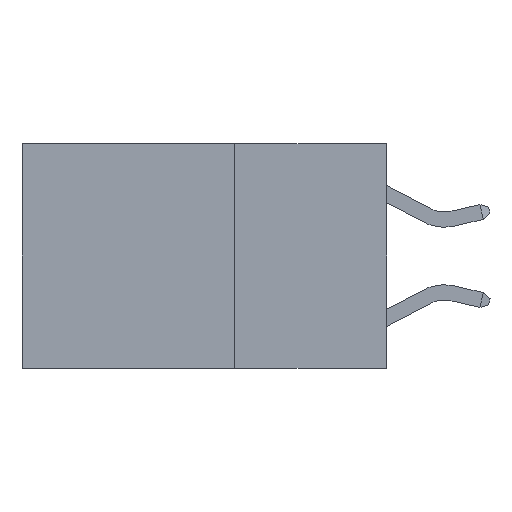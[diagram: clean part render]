
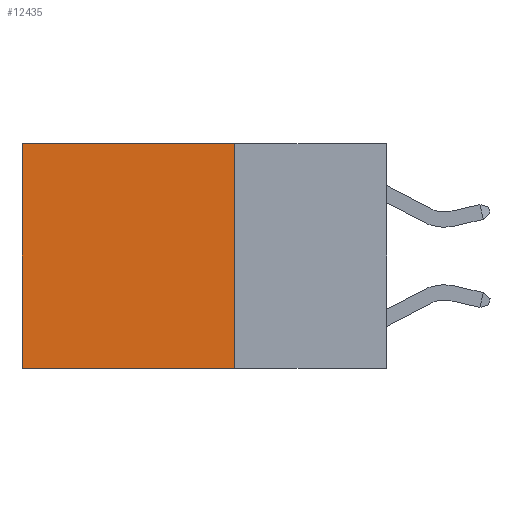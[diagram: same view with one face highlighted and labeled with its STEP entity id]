
A CAD part, left-side view. The second image highlights one B-rep face of the part: STEP entity #12435.
In plain terms, the highlighted planar face has unit normal (-1, 0, 0).
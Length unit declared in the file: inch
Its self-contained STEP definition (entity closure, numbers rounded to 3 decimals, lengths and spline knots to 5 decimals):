
#48 = AXIS2_PLACEMENT_3D ( 'NONE', #2216, #12977, #4648 ) ;
#1903 = VERTEX_POINT ( 'NONE', #17129 ) ;
#2216 = CARTESIAN_POINT ( 'NONE',  ( 0.2625, 0.25, 0. ) ) ;
#2570 = CARTESIAN_POINT ( 'NONE',  ( 0.2625, 0.6, 0. ) ) ;
#4395 = DIRECTION ( 'NONE',  ( 0., 1., 0. ) ) ;
#4520 = VECTOR ( 'NONE', #7856, 39.37008 ) ;
#4601 = CARTESIAN_POINT ( 'NONE',  ( 0.2625, 0.25, -0.37 ) ) ;
#4648 = DIRECTION ( 'NONE',  ( 0., 0., -1. ) ) ;
#4752 = LINE ( 'NONE', #9840, #12570 ) ;
#5280 = LINE ( 'NONE', #2570, #4520 ) ;
#5332 = CARTESIAN_POINT ( 'NONE',  ( 0.2625, 0.6, -0.37 ) ) ;
#5772 = DIRECTION ( 'NONE',  ( 0., 1., 0. ) ) ;
#6567 = EDGE_CURVE ( 'NONE', #1903, #9161, #5280, .T. ) ;
#6581 = EDGE_CURVE ( 'NONE', #9288, #10261, #11991, .T. ) ;
#7680 = CARTESIAN_POINT ( 'NONE',  ( 0.2625, 0.25, 0. ) ) ;
#7856 = DIRECTION ( 'NONE',  ( 0., 0., -1. ) ) ;
#8037 = DIRECTION ( 'NONE',  ( 0., 0., -1. ) ) ;
#8500 = EDGE_CURVE ( 'NONE', #9288, #1903, #4752, .T. ) ;
#8839 = CARTESIAN_POINT ( 'NONE',  ( 0.2625, 0.25, -0.37 ) ) ;
#9161 = VERTEX_POINT ( 'NONE', #5332 ) ;
#9288 = VERTEX_POINT ( 'NONE', #15272 ) ;
#9840 = CARTESIAN_POINT ( 'NONE',  ( 0.2625, 0.25, 0. ) ) ;
#10261 = VERTEX_POINT ( 'NONE', #8839 ) ;
#10986 = ORIENTED_EDGE ( 'NONE', *, *, #6581, .F. ) ;
#11518 = ORIENTED_EDGE ( 'NONE', *, *, #12811, .F. ) ;
#11619 = FACE_OUTER_BOUND ( 'NONE', #13561, .T. ) ;
#11991 = LINE ( 'NONE', #7680, #15112 ) ;
#12435 = ADVANCED_FACE ( 'NONE', ( #11619 ), #17188, .F. ) ;
#12570 = VECTOR ( 'NONE', #4395, 39.37008 ) ;
#12811 = EDGE_CURVE ( 'NONE', #10261, #9161, #15638, .T. ) ;
#12977 = DIRECTION ( 'NONE',  ( 1., 0., 0. ) ) ;
#13561 = EDGE_LOOP ( 'NONE', ( #15117, #11518, #10986, #16286 ) ) ;
#14653 = VECTOR ( 'NONE', #5772, 39.37008 ) ;
#15112 = VECTOR ( 'NONE', #8037, 39.37008 ) ;
#15117 = ORIENTED_EDGE ( 'NONE', *, *, #6567, .T. ) ;
#15272 = CARTESIAN_POINT ( 'NONE',  ( 0.2625, 0.25, 0. ) ) ;
#15638 = LINE ( 'NONE', #4601, #14653 ) ;
#16286 = ORIENTED_EDGE ( 'NONE', *, *, #8500, .T. ) ;
#17129 = CARTESIAN_POINT ( 'NONE',  ( 0.2625, 0.6, 0. ) ) ;
#17188 = PLANE ( 'NONE',  #48 ) ;
